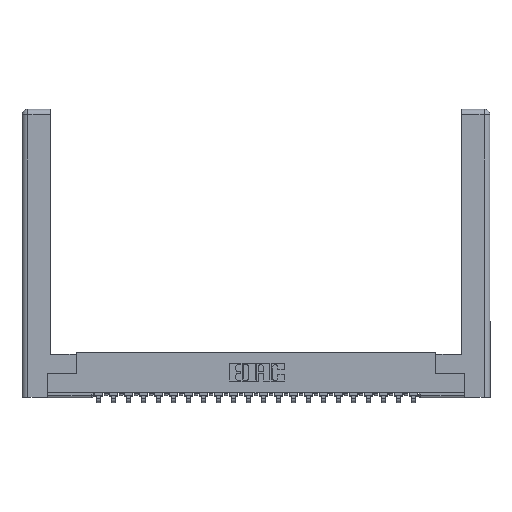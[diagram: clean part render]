
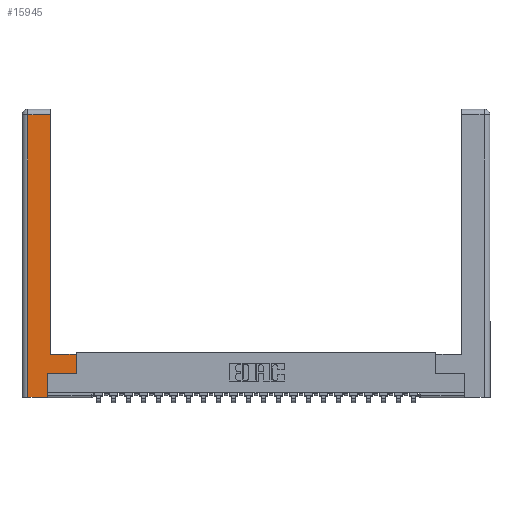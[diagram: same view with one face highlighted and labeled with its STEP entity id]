
A CAD part, top view. The second image highlights one B-rep face of the part: STEP entity #15945.
In plain terms, the highlighted planar face has unit normal (0, 0, 1).
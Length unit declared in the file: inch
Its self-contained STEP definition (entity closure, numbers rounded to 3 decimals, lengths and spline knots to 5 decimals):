
#164 = DIRECTION ( 'NONE',  ( -1., 0., 0. ) ) ;
#331 = LINE ( 'NONE', #5695, #18482 ) ;
#426 = CARTESIAN_POINT ( 'NONE',  ( 0.0615, 2.94, 0. ) ) ;
#529 = CARTESIAN_POINT ( 'NONE',  ( 0.265, 0., 0. ) ) ;
#795 = LINE ( 'NONE', #21641, #1094 ) ;
#1094 = VECTOR ( 'NONE', #23660, 39.37008 ) ;
#1708 = EDGE_CURVE ( 'NONE', #7407, #12393, #795, .T. ) ;
#2302 = CARTESIAN_POINT ( 'NONE',  ( 0.565, 0.245, 0. ) ) ;
#2393 = LINE ( 'NONE', #17954, #4621 ) ;
#2445 = DIRECTION ( 'NONE',  ( 0., 1., 0. ) ) ;
#3214 = CARTESIAN_POINT ( 'NONE',  ( 0.295, 0.45, 0. ) ) ;
#3237 = EDGE_CURVE ( 'NONE', #13965, #20139, #7892, .T. ) ;
#3416 = EDGE_CURVE ( 'NONE', #16188, #9858, #2393, .T. ) ;
#3712 = DIRECTION ( 'NONE',  ( 0., 0., -1. ) ) ;
#3778 = CARTESIAN_POINT ( 'NONE',  ( 0.565, 0.245, 0. ) ) ;
#4052 = VECTOR ( 'NONE', #2445, 39.37008 ) ;
#4070 = LINE ( 'NONE', #9963, #4052 ) ;
#4392 = ORIENTED_EDGE ( 'NONE', *, *, #1708, .T. ) ;
#4621 = VECTOR ( 'NONE', #10406, 39.37008 ) ;
#5084 = LINE ( 'NONE', #3214, #24104 ) ;
#5634 = CARTESIAN_POINT ( 'NONE',  ( 0.265, 0.245, 0. ) ) ;
#5695 = CARTESIAN_POINT ( 'NONE',  ( 0.265, 0., 0. ) ) ;
#6221 = AXIS2_PLACEMENT_3D ( 'NONE', #20794, #3712, #24713 ) ;
#6808 = EDGE_CURVE ( 'NONE', #12393, #16188, #14530, .T. ) ;
#7407 = VERTEX_POINT ( 'NONE', #529 ) ;
#7892 = LINE ( 'NONE', #8013, #24724 ) ;
#8013 = CARTESIAN_POINT ( 'NONE',  ( 0.0615, 2.94, 0. ) ) ;
#8671 = CARTESIAN_POINT ( 'NONE',  ( 0.0615, 0., 0. ) ) ;
#8759 = VECTOR ( 'NONE', #14898, 39.37008 ) ;
#8964 = ORIENTED_EDGE ( 'NONE', *, *, #3237, .T. ) ;
#9360 = FACE_OUTER_BOUND ( 'NONE', #13972, .T. ) ;
#9478 = DIRECTION ( 'NONE',  ( 1., 0., 0. ) ) ;
#9858 = VERTEX_POINT ( 'NONE', #23241 ) ;
#9963 = CARTESIAN_POINT ( 'NONE',  ( 0.295, 3., 0. ) ) ;
#10180 = LINE ( 'NONE', #8671, #17470 ) ;
#10406 = DIRECTION ( 'NONE',  ( 0., 1., 0. ) ) ;
#12393 = VERTEX_POINT ( 'NONE', #5634 ) ;
#12406 = CARTESIAN_POINT ( 'NONE',  ( 0.0615, 0., 0. ) ) ;
#12673 = VERTEX_POINT ( 'NONE', #12406 ) ;
#13965 = VERTEX_POINT ( 'NONE', #21858 ) ;
#13972 = EDGE_LOOP ( 'NONE', ( #23300, #8964, #17374, #16886, #4392, #18609, #24022, #17289 ) ) ;
#14530 = LINE ( 'NONE', #2302, #8759 ) ;
#14847 = EDGE_CURVE ( 'NONE', #20139, #12673, #10180, .T. ) ;
#14886 = DIRECTION ( 'NONE',  ( -1., 0., 0. ) ) ;
#14898 = DIRECTION ( 'NONE',  ( 1., 0., 0. ) ) ;
#15945 = ADVANCED_FACE ( 'NONE', ( #9360 ), #19155, .F. ) ;
#16188 = VERTEX_POINT ( 'NONE', #3778 ) ;
#16738 = CARTESIAN_POINT ( 'NONE',  ( 0.295, 0.45, 0. ) ) ;
#16886 = ORIENTED_EDGE ( 'NONE', *, *, #21669, .T. ) ;
#17289 = ORIENTED_EDGE ( 'NONE', *, *, #21574, .T. ) ;
#17374 = ORIENTED_EDGE ( 'NONE', *, *, #14847, .T. ) ;
#17470 = VECTOR ( 'NONE', #19999, 39.37008 ) ;
#17954 = CARTESIAN_POINT ( 'NONE',  ( 0.565, 0.45, 0. ) ) ;
#18482 = VECTOR ( 'NONE', #9478, 39.37008 ) ;
#18609 = ORIENTED_EDGE ( 'NONE', *, *, #6808, .T. ) ;
#19155 = PLANE ( 'NONE',  #6221 ) ;
#19758 = VERTEX_POINT ( 'NONE', #16738 ) ;
#19999 = DIRECTION ( 'NONE',  ( 0., -1., 0. ) ) ;
#20139 = VERTEX_POINT ( 'NONE', #426 ) ;
#20794 = CARTESIAN_POINT ( 'NONE',  ( 0., 0., 0. ) ) ;
#21574 = EDGE_CURVE ( 'NONE', #9858, #19758, #5084, .T. ) ;
#21641 = CARTESIAN_POINT ( 'NONE',  ( 0.265, 0.245, 0. ) ) ;
#21669 = EDGE_CURVE ( 'NONE', #12673, #7407, #331, .T. ) ;
#21858 = CARTESIAN_POINT ( 'NONE',  ( 0.295, 2.94, 0. ) ) ;
#22785 = EDGE_CURVE ( 'NONE', #19758, #13965, #4070, .T. ) ;
#23241 = CARTESIAN_POINT ( 'NONE',  ( 0.565, 0.45, 0. ) ) ;
#23300 = ORIENTED_EDGE ( 'NONE', *, *, #22785, .T. ) ;
#23660 = DIRECTION ( 'NONE',  ( 0., 1., 0. ) ) ;
#24022 = ORIENTED_EDGE ( 'NONE', *, *, #3416, .T. ) ;
#24104 = VECTOR ( 'NONE', #14886, 39.37008 ) ;
#24713 = DIRECTION ( 'NONE',  ( -1., 0., 0. ) ) ;
#24724 = VECTOR ( 'NONE', #164, 39.37008 ) ;
